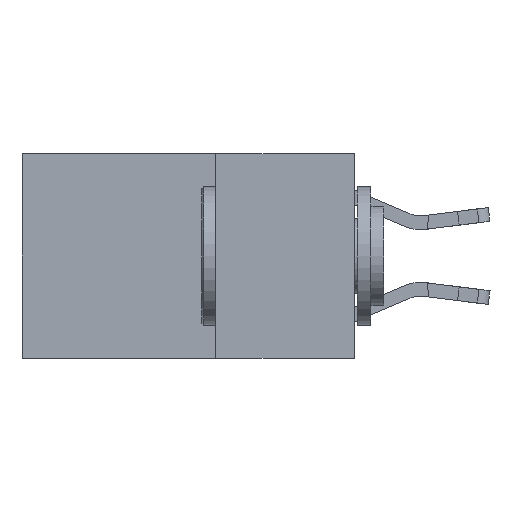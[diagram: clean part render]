
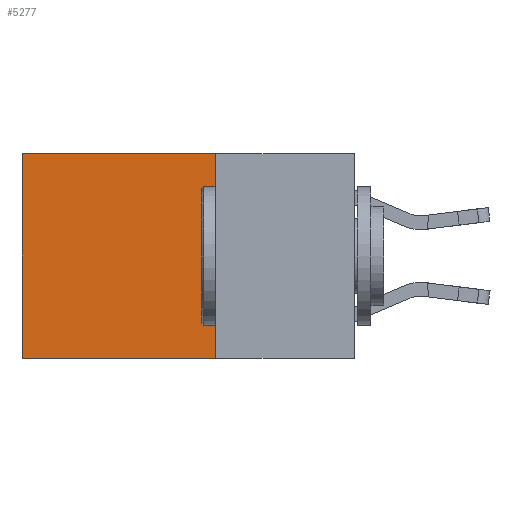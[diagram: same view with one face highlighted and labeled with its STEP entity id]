
A CAD part, left-side view. The second image highlights one B-rep face of the part: STEP entity #5277.
In plain terms, the highlighted planar face has unit normal (-1, 0, 0).
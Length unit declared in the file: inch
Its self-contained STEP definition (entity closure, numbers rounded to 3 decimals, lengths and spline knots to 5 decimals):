
#824 = DIRECTION ( 'NONE',  ( 0., 1., 0. ) ) ;
#1008 = VECTOR ( 'NONE', #5660, 39.37008 ) ;
#1103 = ORIENTED_EDGE ( 'NONE', *, *, #12347, .F. ) ;
#1139 = VECTOR ( 'NONE', #7623, 39.37008 ) ;
#1322 = DIRECTION ( 'NONE',  ( 0., 0., -1. ) ) ;
#1704 = CARTESIAN_POINT ( 'NONE',  ( 0.2625, 0.6, 0. ) ) ;
#2211 = CARTESIAN_POINT ( 'NONE',  ( 0.2625, 0.6, 0. ) ) ;
#2263 = CARTESIAN_POINT ( 'NONE',  ( 0.2625, 0.25, 0. ) ) ;
#2292 = CARTESIAN_POINT ( 'NONE',  ( 0.2625, 0.25, -0.37 ) ) ;
#2367 = VERTEX_POINT ( 'NONE', #2263 ) ;
#2394 = CARTESIAN_POINT ( 'NONE',  ( 0.2625, 0.6, -0.37 ) ) ;
#2428 = CARTESIAN_POINT ( 'NONE',  ( 0.2625, 0.25, -0.37 ) ) ;
#3904 = LINE ( 'NONE', #2428, #1008 ) ;
#4320 = ORIENTED_EDGE ( 'NONE', *, *, #5661, .T. ) ;
#4360 = LINE ( 'NONE', #11777, #1139 ) ;
#4412 = DIRECTION ( 'NONE',  ( 0., 0., -1. ) ) ;
#4535 = CARTESIAN_POINT ( 'NONE',  ( 0.2625, 0.25, 0. ) ) ;
#5277 = ADVANCED_FACE ( 'NONE', ( #11738 ), #12739, .F. ) ;
#5312 = VECTOR ( 'NONE', #4412, 39.37008 ) ;
#5660 = DIRECTION ( 'NONE',  ( 0., 1., 0. ) ) ;
#5661 = EDGE_CURVE ( 'NONE', #2367, #11658, #9659, .T. ) ;
#6531 = VECTOR ( 'NONE', #824, 39.37008 ) ;
#7620 = DIRECTION ( 'NONE',  ( 1., 0., 0. ) ) ;
#7623 = DIRECTION ( 'NONE',  ( 0., 0., -1. ) ) ;
#7656 = VERTEX_POINT ( 'NONE', #2394 ) ;
#8613 = AXIS2_PLACEMENT_3D ( 'NONE', #4535, #7620, #1322 ) ;
#9527 = ORIENTED_EDGE ( 'NONE', *, *, #13217, .F. ) ;
#9542 = VERTEX_POINT ( 'NONE', #2292 ) ;
#9659 = LINE ( 'NONE', #13236, #6531 ) ;
#11192 = LINE ( 'NONE', #2211, #5312 ) ;
#11658 = VERTEX_POINT ( 'NONE', #1704 ) ;
#11738 = FACE_OUTER_BOUND ( 'NONE', #12054, .T. ) ;
#11777 = CARTESIAN_POINT ( 'NONE',  ( 0.2625, 0.25, 0. ) ) ;
#11908 = ORIENTED_EDGE ( 'NONE', *, *, #13092, .T. ) ;
#12054 = EDGE_LOOP ( 'NONE', ( #11908, #1103, #9527, #4320 ) ) ;
#12347 = EDGE_CURVE ( 'NONE', #9542, #7656, #3904, .T. ) ;
#12739 = PLANE ( 'NONE',  #8613 ) ;
#13092 = EDGE_CURVE ( 'NONE', #11658, #7656, #11192, .T. ) ;
#13217 = EDGE_CURVE ( 'NONE', #2367, #9542, #4360, .T. ) ;
#13236 = CARTESIAN_POINT ( 'NONE',  ( 0.2625, 0.25, 0. ) ) ;
